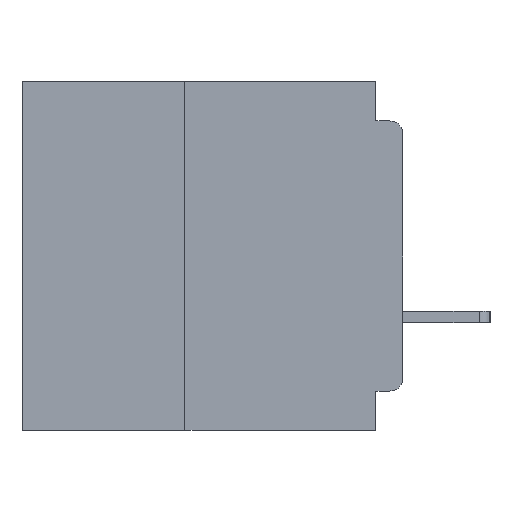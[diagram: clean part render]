
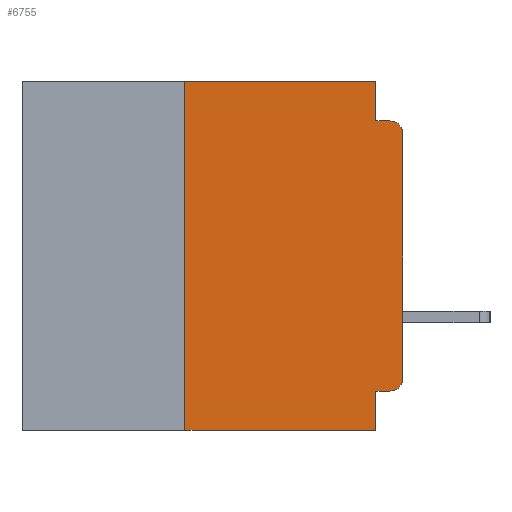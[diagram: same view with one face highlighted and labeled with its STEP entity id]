
A CAD part, left-side view. The second image highlights one B-rep face of the part: STEP entity #6755.
In plain terms, the highlighted planar face has unit normal (-1, 0, 0).
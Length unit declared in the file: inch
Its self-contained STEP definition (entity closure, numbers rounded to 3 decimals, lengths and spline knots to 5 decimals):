
#274 = DIRECTION ( 'NONE',  ( 0., 0., 1. ) ) ;
#320 = DIRECTION ( 'NONE',  ( 1., 0., 0. ) ) ;
#327 = ORIENTED_EDGE ( 'NONE', *, *, #12493, .T. ) ;
#746 = VERTEX_POINT ( 'NONE', #23115 ) ;
#760 = CARTESIAN_POINT ( 'NONE',  ( 0., 0.031, -0.355 ) ) ;
#2117 = LINE ( 'NONE', #5114, #29919 ) ;
#2579 = EDGE_CURVE ( 'NONE', #24153, #25213, #19477, .T. ) ;
#2662 = AXIS2_PLACEMENT_3D ( 'NONE', #16591, #320, #19289 ) ;
#2783 = ORIENTED_EDGE ( 'NONE', *, *, #34330, .T. ) ;
#3053 = EDGE_CURVE ( 'NONE', #19127, #24899, #25711, .T. ) ;
#3186 = ORIENTED_EDGE ( 'NONE', *, *, #3053, .F. ) ;
#3237 = VERTEX_POINT ( 'NONE', #34034 ) ;
#3667 = ORIENTED_EDGE ( 'NONE', *, *, #2579, .T. ) ;
#3698 = CARTESIAN_POINT ( 'NONE',  ( 0., 0.031, -0.045 ) ) ;
#3946 = LINE ( 'NONE', #32518, #11164 ) ;
#4229 = VERTEX_POINT ( 'NONE', #3698 ) ;
#4836 = LINE ( 'NONE', #17377, #18372 ) ;
#5114 = CARTESIAN_POINT ( 'NONE',  ( 0., 0., -0.045 ) ) ;
#5311 = ORIENTED_EDGE ( 'NONE', *, *, #29346, .F. ) ;
#6755 = ADVANCED_FACE ( 'NONE', ( #16691 ), #27232, .F. ) ;
#8412 = EDGE_LOOP ( 'NONE', ( #327, #12837, #21306, #22996, #5311, #3186, #2783, #18014, #17615, #3667 ) ) ;
#8521 = EDGE_CURVE ( 'NONE', #4229, #746, #2117, .T. ) ;
#10122 = CARTESIAN_POINT ( 'NONE',  ( 0., 0.25, -0.4 ) ) ;
#10407 = DIRECTION ( 'NONE',  ( 0., 0., -1. ) ) ;
#10486 = DIRECTION ( 'NONE',  ( -1., 0., 0. ) ) ;
#10563 = CARTESIAN_POINT ( 'NONE',  ( 0., 0.015, -0.34 ) ) ;
#10986 = AXIS2_PLACEMENT_3D ( 'NONE', #10563, #10486, #10407 ) ;
#11164 = VECTOR ( 'NONE', #274, 39.37008 ) ;
#11326 = VERTEX_POINT ( 'NONE', #22590 ) ;
#11381 = DIRECTION ( 'NONE',  ( -1., 0., 0. ) ) ;
#11415 = VECTOR ( 'NONE', #12164, 39.37008 ) ;
#11693 = EDGE_CURVE ( 'NONE', #24153, #17589, #12061, .T. ) ;
#11900 = CARTESIAN_POINT ( 'NONE',  ( 0., 0.031, -0.4 ) ) ;
#12048 = CIRCLE ( 'NONE', #23344, 0.015 ) ;
#12061 = LINE ( 'NONE', #32082, #20097 ) ;
#12075 = EDGE_CURVE ( 'NONE', #30548, #4229, #4836, .T. ) ;
#12164 = DIRECTION ( 'NONE',  ( 0., 0., 1. ) ) ;
#12493 = EDGE_CURVE ( 'NONE', #25213, #3237, #3946, .T. ) ;
#12771 = LINE ( 'NONE', #31120, #17421 ) ;
#12837 = ORIENTED_EDGE ( 'NONE', *, *, #30414, .T. ) ;
#13374 = DIRECTION ( 'NONE',  ( 0., 1., 0. ) ) ;
#13425 = CARTESIAN_POINT ( 'NONE',  ( 0., 0.015, -0.355 ) ) ;
#14187 = DIRECTION ( 'NONE',  ( 0., -1., 0. ) ) ;
#14304 = CARTESIAN_POINT ( 'NONE',  ( 0., 0.437, 0. ) ) ;
#14566 = CARTESIAN_POINT ( 'NONE',  ( 0., 0.25, 0. ) ) ;
#16591 = CARTESIAN_POINT ( 'NONE',  ( 0., 0.437, 0. ) ) ;
#16691 = FACE_OUTER_BOUND ( 'NONE', #8412, .T. ) ;
#17278 = CARTESIAN_POINT ( 'NONE',  ( 0., 0.031, 0. ) ) ;
#17377 = CARTESIAN_POINT ( 'NONE',  ( 0., 0.031, 0. ) ) ;
#17421 = VECTOR ( 'NONE', #33754, 39.37008 ) ;
#17589 = VERTEX_POINT ( 'NONE', #760 ) ;
#17615 = ORIENTED_EDGE ( 'NONE', *, *, #11693, .F. ) ;
#18014 = ORIENTED_EDGE ( 'NONE', *, *, #25514, .F. ) ;
#18101 = CARTESIAN_POINT ( 'NONE',  ( 0., 0.25, -0.4 ) ) ;
#18372 = VECTOR ( 'NONE', #22694, 39.37008 ) ;
#19127 = VERTEX_POINT ( 'NONE', #18101 ) ;
#19289 = DIRECTION ( 'NONE',  ( 0., 0., -1. ) ) ;
#19477 = CIRCLE ( 'NONE', #10986, 0.015 ) ;
#20097 = VECTOR ( 'NONE', #13374, 39.37008 ) ;
#20888 = LINE ( 'NONE', #11900, #21749 ) ;
#21306 = ORIENTED_EDGE ( 'NONE', *, *, #8521, .F. ) ;
#21438 = VECTOR ( 'NONE', #14187, 39.37008 ) ;
#21749 = VECTOR ( 'NONE', #33300, 39.37008 ) ;
#22590 = CARTESIAN_POINT ( 'NONE',  ( 0., 0.031, -0.4 ) ) ;
#22694 = DIRECTION ( 'NONE',  ( 0., 0., -1. ) ) ;
#22996 = ORIENTED_EDGE ( 'NONE', *, *, #12075, .F. ) ;
#23115 = CARTESIAN_POINT ( 'NONE',  ( 0., 0.015, -0.045 ) ) ;
#23344 = AXIS2_PLACEMENT_3D ( 'NONE', #27457, #11381, #30142 ) ;
#23962 = CARTESIAN_POINT ( 'NONE',  ( 0., 0., -0.34 ) ) ;
#24153 = VERTEX_POINT ( 'NONE', #13425 ) ;
#24899 = VERTEX_POINT ( 'NONE', #14566 ) ;
#25213 = VERTEX_POINT ( 'NONE', #23962 ) ;
#25514 = EDGE_CURVE ( 'NONE', #17589, #11326, #20888, .T. ) ;
#25711 = LINE ( 'NONE', #10122, #11415 ) ;
#27232 = PLANE ( 'NONE',  #2662 ) ;
#27457 = CARTESIAN_POINT ( 'NONE',  ( 0., 0.015, -0.06 ) ) ;
#29346 = EDGE_CURVE ( 'NONE', #24899, #30548, #34707, .T. ) ;
#29919 = VECTOR ( 'NONE', #34635, 39.37008 ) ;
#30142 = DIRECTION ( 'NONE',  ( 0., 0., -1. ) ) ;
#30414 = EDGE_CURVE ( 'NONE', #3237, #746, #12048, .T. ) ;
#30548 = VERTEX_POINT ( 'NONE', #17278 ) ;
#31120 = CARTESIAN_POINT ( 'NONE',  ( 0., 0.437, -0.4 ) ) ;
#32082 = CARTESIAN_POINT ( 'NONE',  ( 0., 0., -0.355 ) ) ;
#32518 = CARTESIAN_POINT ( 'NONE',  ( 0., 0., 0. ) ) ;
#33300 = DIRECTION ( 'NONE',  ( 0., 0., -1. ) ) ;
#33754 = DIRECTION ( 'NONE',  ( 0., -1., 0. ) ) ;
#34034 = CARTESIAN_POINT ( 'NONE',  ( 0., 0., -0.06 ) ) ;
#34330 = EDGE_CURVE ( 'NONE', #19127, #11326, #12771, .T. ) ;
#34635 = DIRECTION ( 'NONE',  ( 0., -1., 0. ) ) ;
#34707 = LINE ( 'NONE', #14304, #21438 ) ;
